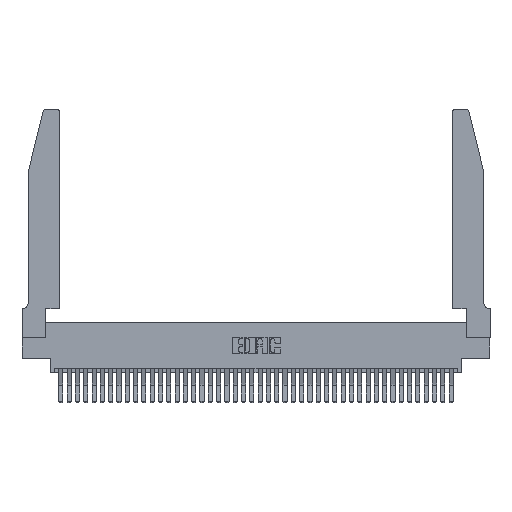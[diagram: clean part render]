
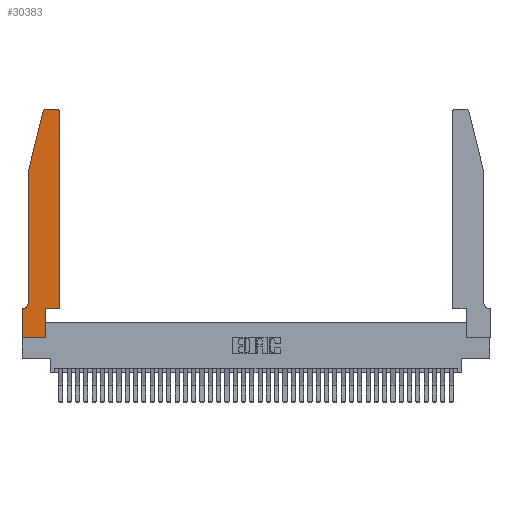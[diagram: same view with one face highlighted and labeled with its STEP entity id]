
A CAD part, top view. The second image highlights one B-rep face of the part: STEP entity #30383.
In plain terms, the highlighted planar face has unit normal (0, 0, 1).
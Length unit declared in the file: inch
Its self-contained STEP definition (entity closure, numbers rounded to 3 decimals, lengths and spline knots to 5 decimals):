
#259 = CARTESIAN_POINT ( 'NONE',  ( 0.2865, 0.35, 0.37 ) ) ;
#356 = ORIENTED_EDGE ( 'NONE', *, *, #16009, .T. ) ;
#478 = LINE ( 'NONE', #16915, #8305 ) ;
#583 = EDGE_CURVE ( 'NONE', #25812, #27283, #35382, .T. ) ;
#756 = FACE_OUTER_BOUND ( 'NONE', #26050, .T. ) ;
#992 = LINE ( 'NONE', #22432, #25938 ) ;
#1462 = DIRECTION ( 'NONE',  ( 0., 0., -1. ) ) ;
#1470 = EDGE_CURVE ( 'NONE', #11445, #25812, #19285, .T. ) ;
#2531 = CARTESIAN_POINT ( 'NONE',  ( 0.0755, 2., 0.37 ) ) ;
#3716 = CARTESIAN_POINT ( 'NONE',  ( 0., 0.35, 0.37 ) ) ;
#4184 = ORIENTED_EDGE ( 'NONE', *, *, #20754, .T. ) ;
#4319 = VERTEX_POINT ( 'NONE', #3716 ) ;
#4345 = EDGE_CURVE ( 'NONE', #27283, #12877, #36631, .T. ) ;
#4999 = DIRECTION ( 'NONE',  ( 1., 0., 0. ) ) ;
#5157 = CARTESIAN_POINT ( 'NONE',  ( 0.4505, 0.35, 0.37 ) ) ;
#5483 = VERTEX_POINT ( 'NONE', #29346 ) ;
#6966 = AXIS2_PLACEMENT_3D ( 'NONE', #21009, #1462, #24233 ) ;
#7318 = CARTESIAN_POINT ( 'NONE',  ( 0.4205, 2.72, 0.37 ) ) ;
#7681 = ORIENTED_EDGE ( 'NONE', *, *, #583, .T. ) ;
#7806 = VECTOR ( 'NONE', #30008, 39.37008 ) ;
#8305 = VECTOR ( 'NONE', #20126, 39.37008 ) ;
#8398 = LINE ( 'NONE', #5157, #40513 ) ;
#8476 = EDGE_CURVE ( 'NONE', #4319, #33402, #24986, .T. ) ;
#8913 = EDGE_CURVE ( 'NONE', #12877, #28190, #992, .T. ) ;
#9268 = ORIENTED_EDGE ( 'NONE', *, *, #8476, .T. ) ;
#9687 = VERTEX_POINT ( 'NONE', #13165 ) ;
#9951 = CARTESIAN_POINT ( 'NONE',  ( 0.284, 2.75, 0.37 ) ) ;
#10417 = CIRCLE ( 'NONE', #6966, 0.07 ) ;
#10629 = DIRECTION ( 'NONE',  ( 1., 0., 0. ) ) ;
#10642 = CARTESIAN_POINT ( 'NONE',  ( 0.0755, 2., 0.37 ) ) ;
#11017 = ORIENTED_EDGE ( 'NONE', *, *, #30789, .T. ) ;
#11197 = VECTOR ( 'NONE', #14236, 39.37008 ) ;
#11445 = VERTEX_POINT ( 'NONE', #22301 ) ;
#11478 = CARTESIAN_POINT ( 'NONE',  ( 0., 0.35, 0.37 ) ) ;
#11548 = CARTESIAN_POINT ( 'NONE',  ( 0.25487, 2.72718, 0.37 ) ) ;
#11860 = DIRECTION ( 'NONE',  ( 0., 0., 1. ) ) ;
#12877 = VERTEX_POINT ( 'NONE', #2531 ) ;
#12916 = CARTESIAN_POINT ( 'NONE',  ( 0.2605, 2.75, 0.37 ) ) ;
#12984 = VERTEX_POINT ( 'NONE', #32089 ) ;
#13165 = CARTESIAN_POINT ( 'NONE',  ( 0.2865, 0., 0.37 ) ) ;
#13763 = EDGE_CURVE ( 'NONE', #25860, #4319, #478, .T. ) ;
#14236 = DIRECTION ( 'NONE',  ( 0., 1., 0. ) ) ;
#14285 = ORIENTED_EDGE ( 'NONE', *, *, #8913, .T. ) ;
#14904 = ORIENTED_EDGE ( 'NONE', *, *, #30072, .T. ) ;
#15743 = VECTOR ( 'NONE', #29040, 39.37008 ) ;
#16009 = EDGE_CURVE ( 'NONE', #5483, #12984, #36761, .T. ) ;
#16915 = CARTESIAN_POINT ( 'NONE',  ( 0.0755, 0.35, 0.37 ) ) ;
#19147 = ORIENTED_EDGE ( 'NONE', *, *, #1470, .T. ) ;
#19285 = LINE ( 'NONE', #12916, #36298 ) ;
#20126 = DIRECTION ( 'NONE',  ( -1., 0., 0. ) ) ;
#20613 = VECTOR ( 'NONE', #33072, 39.37008 ) ;
#20679 = CIRCLE ( 'NONE', #28719, 0.03 ) ;
#20754 = EDGE_CURVE ( 'NONE', #12984, #11445, #20679, .T. ) ;
#21009 = CARTESIAN_POINT ( 'NONE',  ( 0.0055, 0.42, 0.37 ) ) ;
#21165 = PLANE ( 'NONE',  #28407 ) ;
#22301 = CARTESIAN_POINT ( 'NONE',  ( 0.4205, 2.75, 0.37 ) ) ;
#22432 = CARTESIAN_POINT ( 'NONE',  ( 0.0755, 2., 0.37 ) ) ;
#22592 = CARTESIAN_POINT ( 'NONE',  ( 0., 0., 0.37 ) ) ;
#22707 = ORIENTED_EDGE ( 'NONE', *, *, #26593, .T. ) ;
#23080 = DIRECTION ( 'NONE',  ( 0., 1., 0. ) ) ;
#24233 = DIRECTION ( 'NONE',  ( -1., 0., 0. ) ) ;
#24387 = DIRECTION ( 'NONE',  ( 0., 0., 1. ) ) ;
#24986 = LINE ( 'NONE', #26803, #7806 ) ;
#25656 = DIRECTION ( 'NONE',  ( 0., -1., 0. ) ) ;
#25812 = VERTEX_POINT ( 'NONE', #9951 ) ;
#25860 = VERTEX_POINT ( 'NONE', #26238 ) ;
#25938 = VECTOR ( 'NONE', #25656, 39.37008 ) ;
#26050 = EDGE_LOOP ( 'NONE', ( #19147, #7681, #34501, #14285, #22707, #29875, #9268, #14904, #11017, #34194, #356, #4184 ) ) ;
#26117 = AXIS2_PLACEMENT_3D ( 'NONE', #31080, #11860, #34284 ) ;
#26180 = EDGE_CURVE ( 'NONE', #27316, #5483, #8398, .T. ) ;
#26238 = CARTESIAN_POINT ( 'NONE',  ( 0.0055, 0.35, 0.37 ) ) ;
#26593 = EDGE_CURVE ( 'NONE', #28190, #25860, #10417, .T. ) ;
#26682 = LINE ( 'NONE', #259, #36182 ) ;
#26803 = CARTESIAN_POINT ( 'NONE',  ( 0., 0., 0.37 ) ) ;
#27283 = VERTEX_POINT ( 'NONE', #11548 ) ;
#27316 = VERTEX_POINT ( 'NONE', #40353 ) ;
#28190 = VERTEX_POINT ( 'NONE', #31791 ) ;
#28407 = AXIS2_PLACEMENT_3D ( 'NONE', #11478, #24387, #4999 ) ;
#28719 = AXIS2_PLACEMENT_3D ( 'NONE', #7318, #29842, #10629 ) ;
#29040 = DIRECTION ( 'NONE',  ( 1., 0., 0. ) ) ;
#29346 = CARTESIAN_POINT ( 'NONE',  ( 0.4505, 0.35, 0.37 ) ) ;
#29842 = DIRECTION ( 'NONE',  ( 0., 0., 1. ) ) ;
#29875 = ORIENTED_EDGE ( 'NONE', *, *, #13763, .T. ) ;
#30008 = DIRECTION ( 'NONE',  ( 0., -1., 0. ) ) ;
#30072 = EDGE_CURVE ( 'NONE', #33402, #9687, #31763, .T. ) ;
#30205 = CARTESIAN_POINT ( 'NONE',  ( 0.4505, 0.35, 0.37 ) ) ;
#30383 = ADVANCED_FACE ( 'NONE', ( #756 ), #21165, .T. ) ;
#30789 = EDGE_CURVE ( 'NONE', #9687, #27316, #26682, .T. ) ;
#30968 = DIRECTION ( 'NONE',  ( 1., 0., 0. ) ) ;
#31080 = CARTESIAN_POINT ( 'NONE',  ( 0.284, 2.72, 0.37 ) ) ;
#31763 = LINE ( 'NONE', #22592, #15743 ) ;
#31791 = CARTESIAN_POINT ( 'NONE',  ( 0.0755, 0.42, 0.37 ) ) ;
#32089 = CARTESIAN_POINT ( 'NONE',  ( 0.4505, 2.72, 0.37 ) ) ;
#33072 = DIRECTION ( 'NONE',  ( -0.239, -0.971, 0. ) ) ;
#33402 = VERTEX_POINT ( 'NONE', #34717 ) ;
#34194 = ORIENTED_EDGE ( 'NONE', *, *, #26180, .T. ) ;
#34284 = DIRECTION ( 'NONE',  ( 1., 0., 0. ) ) ;
#34501 = ORIENTED_EDGE ( 'NONE', *, *, #4345, .T. ) ;
#34717 = CARTESIAN_POINT ( 'NONE',  ( 0., 0., 0.37 ) ) ;
#35356 = DIRECTION ( 'NONE',  ( -1., 0., 0. ) ) ;
#35382 = CIRCLE ( 'NONE', #26117, 0.03 ) ;
#36182 = VECTOR ( 'NONE', #23080, 39.37008 ) ;
#36298 = VECTOR ( 'NONE', #35356, 39.37008 ) ;
#36631 = LINE ( 'NONE', #10642, #20613 ) ;
#36761 = LINE ( 'NONE', #30205, #11197 ) ;
#40353 = CARTESIAN_POINT ( 'NONE',  ( 0.2865, 0.35, 0.37 ) ) ;
#40513 = VECTOR ( 'NONE', #30968, 39.37008 ) ;
